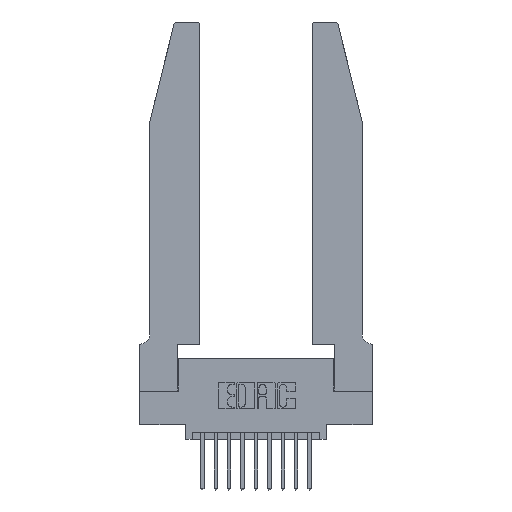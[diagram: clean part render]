
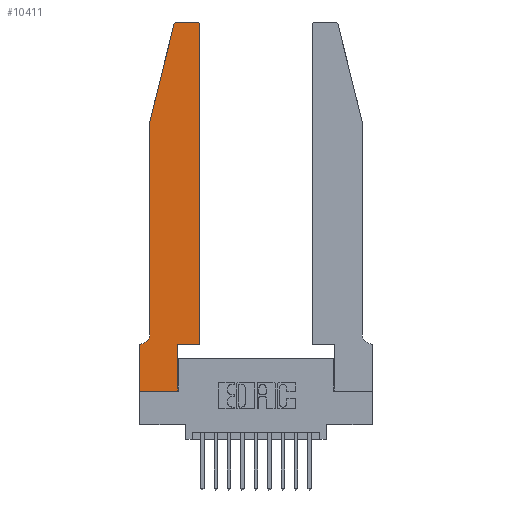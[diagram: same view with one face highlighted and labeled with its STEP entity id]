
A CAD part, top view. The second image highlights one B-rep face of the part: STEP entity #10411.
In plain terms, the highlighted planar face has unit normal (0, 0, 1).
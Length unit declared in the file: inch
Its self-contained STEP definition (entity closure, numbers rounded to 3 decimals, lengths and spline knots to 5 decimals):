
#166 = CARTESIAN_POINT ( 'NONE',  ( 0.284, 2.75, 0.37 ) ) ;
#341 = DIRECTION ( 'NONE',  ( 1., 0., 0. ) ) ;
#508 = CIRCLE ( 'NONE', #597, 0.07 ) ;
#597 = AXIS2_PLACEMENT_3D ( 'NONE', #4808, #7267, #9805 ) ;
#686 = EDGE_CURVE ( 'NONE', #1459, #8674, #14800, .T. ) ;
#720 = LINE ( 'NONE', #8222, #12015 ) ;
#929 = CARTESIAN_POINT ( 'NONE',  ( 0.2605, 2.75, 0.37 ) ) ;
#1313 = DIRECTION ( 'NONE',  ( 1., 0., 0. ) ) ;
#1399 = AXIS2_PLACEMENT_3D ( 'NONE', #9972, #2403, #8769 ) ;
#1459 = VERTEX_POINT ( 'NONE', #5607 ) ;
#1846 = VECTOR ( 'NONE', #11052, 39.37008 ) ;
#1900 = ORIENTED_EDGE ( 'NONE', *, *, #4485, .T. ) ;
#2359 = VERTEX_POINT ( 'NONE', #9525 ) ;
#2377 = CARTESIAN_POINT ( 'NONE',  ( 0., 0., 0.37 ) ) ;
#2403 = DIRECTION ( 'NONE',  ( 0., 0., 1. ) ) ;
#2772 = ORIENTED_EDGE ( 'NONE', *, *, #686, .T. ) ;
#2925 = FACE_OUTER_BOUND ( 'NONE', #12892, .T. ) ;
#3113 = CARTESIAN_POINT ( 'NONE',  ( 0.0755, 2., 0.37 ) ) ;
#3227 = DIRECTION ( 'NONE',  ( -1., 0., 0. ) ) ;
#3377 = AXIS2_PLACEMENT_3D ( 'NONE', #14079, #12830, #4090 ) ;
#3721 = ORIENTED_EDGE ( 'NONE', *, *, #9327, .T. ) ;
#3763 = CARTESIAN_POINT ( 'NONE',  ( 0., 0., 0.37 ) ) ;
#3828 = EDGE_CURVE ( 'NONE', #9663, #8733, #508, .T. ) ;
#4090 = DIRECTION ( 'NONE',  ( 1., 0., 0. ) ) ;
#4324 = VECTOR ( 'NONE', #12022, 39.37008 ) ;
#4364 = CARTESIAN_POINT ( 'NONE',  ( 0.4505, 0.35, 0.37 ) ) ;
#4485 = EDGE_CURVE ( 'NONE', #2359, #8547, #9585, .T. ) ;
#4517 = CARTESIAN_POINT ( 'NONE',  ( 0.4505, 0.35, 0.37 ) ) ;
#4707 = EDGE_CURVE ( 'NONE', #15966, #8014, #9570, .T. ) ;
#4808 = CARTESIAN_POINT ( 'NONE',  ( 0.0055, 0.42, 0.37 ) ) ;
#5091 = AXIS2_PLACEMENT_3D ( 'NONE', #10523, #15611, #341 ) ;
#5367 = EDGE_CURVE ( 'NONE', #8014, #8787, #9755, .T. ) ;
#5607 = CARTESIAN_POINT ( 'NONE',  ( 0., 0.35, 0.37 ) ) ;
#5766 = EDGE_CURVE ( 'NONE', #6604, #14562, #7631, .T. ) ;
#5840 = LINE ( 'NONE', #3763, #16366 ) ;
#6120 = CARTESIAN_POINT ( 'NONE',  ( 0.2865, 0.35, 0.37 ) ) ;
#6145 = ORIENTED_EDGE ( 'NONE', *, *, #11274, .T. ) ;
#6245 = ORIENTED_EDGE ( 'NONE', *, *, #13983, .T. ) ;
#6479 = CARTESIAN_POINT ( 'NONE',  ( 0.0055, 0.35, 0.37 ) ) ;
#6604 = VERTEX_POINT ( 'NONE', #16059 ) ;
#6647 = VECTOR ( 'NONE', #9083, 39.37008 ) ;
#6710 = ORIENTED_EDGE ( 'NONE', *, *, #15975, .T. ) ;
#6810 = ORIENTED_EDGE ( 'NONE', *, *, #5367, .T. ) ;
#7145 = DIRECTION ( 'NONE',  ( 1., 0., 0. ) ) ;
#7267 = DIRECTION ( 'NONE',  ( 0., 0., -1. ) ) ;
#7486 = ORIENTED_EDGE ( 'NONE', *, *, #5766, .T. ) ;
#7540 = PLANE ( 'NONE',  #1399 ) ;
#7631 = LINE ( 'NONE', #15384, #6647 ) ;
#8014 = VERTEX_POINT ( 'NONE', #14313 ) ;
#8131 = CARTESIAN_POINT ( 'NONE',  ( 0.0755, 2., 0.37 ) ) ;
#8222 = CARTESIAN_POINT ( 'NONE',  ( 0.0755, 0.35, 0.37 ) ) ;
#8547 = VERTEX_POINT ( 'NONE', #6120 ) ;
#8674 = VERTEX_POINT ( 'NONE', #13965 ) ;
#8701 = VECTOR ( 'NONE', #16340, 39.37008 ) ;
#8733 = VERTEX_POINT ( 'NONE', #6479 ) ;
#8769 = DIRECTION ( 'NONE',  ( 1., 0., 0. ) ) ;
#8787 = VERTEX_POINT ( 'NONE', #166 ) ;
#8842 = VERTEX_POINT ( 'NONE', #13006 ) ;
#8866 = LINE ( 'NONE', #4517, #12020 ) ;
#9083 = DIRECTION ( 'NONE',  ( -0.239, -0.971, 0. ) ) ;
#9290 = LINE ( 'NONE', #8131, #16213 ) ;
#9309 = EDGE_CURVE ( 'NONE', #8842, #15966, #13620, .T. ) ;
#9327 = EDGE_CURVE ( 'NONE', #8787, #6604, #11659, .T. ) ;
#9525 = CARTESIAN_POINT ( 'NONE',  ( 0.2865, 0., 0.37 ) ) ;
#9570 = CIRCLE ( 'NONE', #3377, 0.03 ) ;
#9585 = LINE ( 'NONE', #11793, #9975 ) ;
#9663 = VERTEX_POINT ( 'NONE', #12000 ) ;
#9755 = LINE ( 'NONE', #929, #1846 ) ;
#9805 = DIRECTION ( 'NONE',  ( -1., 0., 0. ) ) ;
#9972 = CARTESIAN_POINT ( 'NONE',  ( 0., 0.35, 0.37 ) ) ;
#9975 = VECTOR ( 'NONE', #13005, 39.37008 ) ;
#10411 = ADVANCED_FACE ( 'NONE', ( #2925 ), #7540, .T. ) ;
#10523 = CARTESIAN_POINT ( 'NONE',  ( 0.284, 2.72, 0.37 ) ) ;
#10592 = EDGE_CURVE ( 'NONE', #8733, #1459, #720, .T. ) ;
#10655 = DIRECTION ( 'NONE',  ( 0., -1., 0. ) ) ;
#10686 = ORIENTED_EDGE ( 'NONE', *, *, #3828, .T. ) ;
#11052 = DIRECTION ( 'NONE',  ( -1., 0., 0. ) ) ;
#11274 = EDGE_CURVE ( 'NONE', #8547, #8842, #8866, .T. ) ;
#11381 = CARTESIAN_POINT ( 'NONE',  ( 0.4505, 2.72, 0.37 ) ) ;
#11659 = CIRCLE ( 'NONE', #5091, 0.03 ) ;
#11793 = CARTESIAN_POINT ( 'NONE',  ( 0.2865, 0.35, 0.37 ) ) ;
#12000 = CARTESIAN_POINT ( 'NONE',  ( 0.0755, 0.42, 0.37 ) ) ;
#12015 = VECTOR ( 'NONE', #3227, 39.37008 ) ;
#12020 = VECTOR ( 'NONE', #7145, 39.37008 ) ;
#12022 = DIRECTION ( 'NONE',  ( 0., 1., 0. ) ) ;
#12689 = ORIENTED_EDGE ( 'NONE', *, *, #4707, .T. ) ;
#12830 = DIRECTION ( 'NONE',  ( 0., 0., 1. ) ) ;
#12892 = EDGE_LOOP ( 'NONE', ( #6810, #3721, #7486, #6245, #10686, #15022, #2772, #6710, #1900, #6145, #14274, #12689 ) ) ;
#13005 = DIRECTION ( 'NONE',  ( 0., 1., 0. ) ) ;
#13006 = CARTESIAN_POINT ( 'NONE',  ( 0.4505, 0.35, 0.37 ) ) ;
#13620 = LINE ( 'NONE', #4364, #4324 ) ;
#13965 = CARTESIAN_POINT ( 'NONE',  ( 0., 0., 0.37 ) ) ;
#13983 = EDGE_CURVE ( 'NONE', #14562, #9663, #9290, .T. ) ;
#14079 = CARTESIAN_POINT ( 'NONE',  ( 0.4205, 2.72, 0.37 ) ) ;
#14274 = ORIENTED_EDGE ( 'NONE', *, *, #9309, .T. ) ;
#14313 = CARTESIAN_POINT ( 'NONE',  ( 0.4205, 2.75, 0.37 ) ) ;
#14562 = VERTEX_POINT ( 'NONE', #3113 ) ;
#14800 = LINE ( 'NONE', #2377, #8701 ) ;
#15022 = ORIENTED_EDGE ( 'NONE', *, *, #10592, .T. ) ;
#15384 = CARTESIAN_POINT ( 'NONE',  ( 0.0755, 2., 0.37 ) ) ;
#15611 = DIRECTION ( 'NONE',  ( 0., 0., 1. ) ) ;
#15966 = VERTEX_POINT ( 'NONE', #11381 ) ;
#15975 = EDGE_CURVE ( 'NONE', #8674, #2359, #5840, .T. ) ;
#16059 = CARTESIAN_POINT ( 'NONE',  ( 0.25487, 2.72718, 0.37 ) ) ;
#16213 = VECTOR ( 'NONE', #10655, 39.37008 ) ;
#16340 = DIRECTION ( 'NONE',  ( 0., -1., 0. ) ) ;
#16366 = VECTOR ( 'NONE', #1313, 39.37008 ) ;
